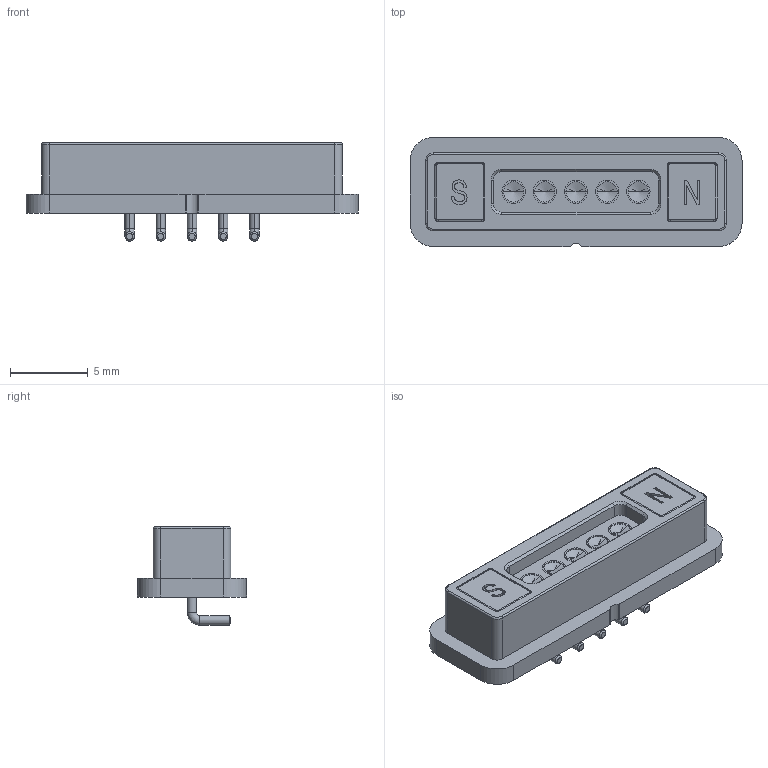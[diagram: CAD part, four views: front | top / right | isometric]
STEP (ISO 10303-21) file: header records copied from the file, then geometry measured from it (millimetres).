
FILE_DESCRIPTION (( 'STEP AP214' ), '1' );
FILE_NAME ('686J0521350110E.STEP', '2023-04-13T19:07:18', ( '' ), ( '' ), 'SwSTEP 2.0', 'SolidWorks 2020', '' );
FILE_SCHEMA (( 'AUTOMOTIVE_DESIGN' ));
Length unit declared in the file: millimetre
Products named in the file (1): 686J0521350110E
Bounding box: 21.3 x 7 x 6.3 mm (x, y, z)
Volume: 433.1 mm3; surface area: 697.3 mm2
Topology: 6 solids, 8 shells, 276 faces, 625 edges, 380 vertices
Faces by surface type: cylinder 111, plane 95, cone 26, torus 24, bspline 20
Entity records: 10993 total; most frequent: CARTESIAN_POINT 2192, DIRECTION 1368, ORIENTED_EDGE 1230, EDGE_CURVE 615, AXIS2_PLACEMENT_3D 524, VERTEX_POINT 380, LINE 320, VECTOR 320
